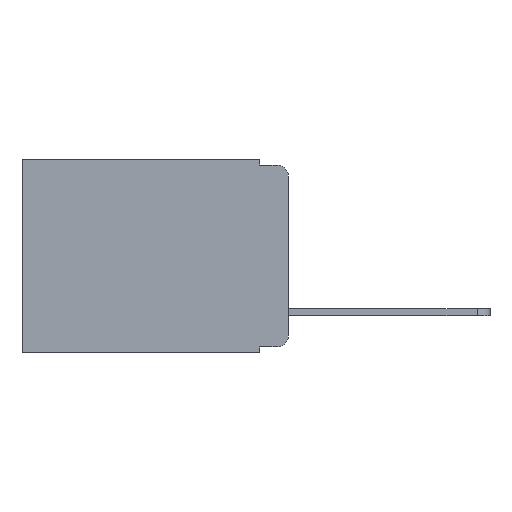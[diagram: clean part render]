
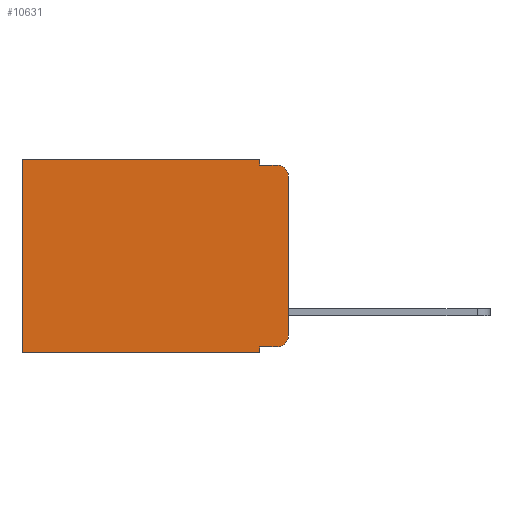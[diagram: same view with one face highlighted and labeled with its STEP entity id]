
A CAD part, left-side view. The second image highlights one B-rep face of the part: STEP entity #10631.
In plain terms, the highlighted planar face has unit normal (-1, 0, 0).
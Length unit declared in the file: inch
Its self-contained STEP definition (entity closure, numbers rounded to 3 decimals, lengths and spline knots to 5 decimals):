
#285 = DIRECTION ( 'NONE',  ( 0., 0., -1. ) ) ;
#680 = VECTOR ( 'NONE', #7780, 39.37008 ) ;
#1125 = ORIENTED_EDGE ( 'NONE', *, *, #13841, .T. ) ;
#1165 = VERTEX_POINT ( 'NONE', #4860 ) ;
#1272 = DIRECTION ( 'NONE',  ( 0., 0., -1. ) ) ;
#1438 = CARTESIAN_POINT ( 'NONE',  ( 0.298, 0.051, 0. ) ) ;
#1664 = VERTEX_POINT ( 'NONE', #4927 ) ;
#1966 = EDGE_LOOP ( 'NONE', ( #3705, #6823, #3880, #10232, #13664, #1125, #7923, #10960, #8287, #14346 ) ) ;
#2559 = DIRECTION ( 'NONE',  ( 1., 0., 0. ) ) ;
#2642 = DIRECTION ( 'NONE',  ( 0., 1., 0. ) ) ;
#3253 = LINE ( 'NONE', #14003, #12418 ) ;
#3318 = EDGE_CURVE ( 'NONE', #4113, #7942, #11637, .T. ) ;
#3705 = ORIENTED_EDGE ( 'NONE', *, *, #4437, .F. ) ;
#3880 = ORIENTED_EDGE ( 'NONE', *, *, #14892, .F. ) ;
#4113 = VERTEX_POINT ( 'NONE', #10030 ) ;
#4163 = EDGE_CURVE ( 'NONE', #7310, #6095, #6894, .T. ) ;
#4204 = VERTEX_POINT ( 'NONE', #15331 ) ;
#4225 = CARTESIAN_POINT ( 'NONE',  ( 0.298, 0., -0.313 ) ) ;
#4250 = CARTESIAN_POINT ( 'NONE',  ( 0.298, 0., -0.03 ) ) ;
#4437 = EDGE_CURVE ( 'NONE', #7310, #7942, #11784, .T. ) ;
#4533 = EDGE_CURVE ( 'NONE', #11388, #5750, #8340, .T. ) ;
#4670 = LINE ( 'NONE', #15644, #13327 ) ;
#4860 = CARTESIAN_POINT ( 'NONE',  ( 0.298, 0.051, -0.01 ) ) ;
#4927 = CARTESIAN_POINT ( 'NONE',  ( 0.298, 0.051, -0.343 ) ) ;
#4986 = CARTESIAN_POINT ( 'NONE',  ( 0.298, 0.02, -0.313 ) ) ;
#5750 = VERTEX_POINT ( 'NONE', #5873 ) ;
#5873 = CARTESIAN_POINT ( 'NONE',  ( 0.298, 0.473, 0. ) ) ;
#6095 = VERTEX_POINT ( 'NONE', #8014 ) ;
#6322 = LINE ( 'NONE', #11859, #15131 ) ;
#6343 = DIRECTION ( 'NONE',  ( -1., 0., 0. ) ) ;
#6374 = PLANE ( 'NONE',  #6998 ) ;
#6377 = CARTESIAN_POINT ( 'NONE',  ( 0.298, 0., 0. ) ) ;
#6823 = ORIENTED_EDGE ( 'NONE', *, *, #4163, .T. ) ;
#6894 = CIRCLE ( 'NONE', #10282, 0.02 ) ;
#6941 = DIRECTION ( 'NONE',  ( 0., 0., -1. ) ) ;
#6998 = AXIS2_PLACEMENT_3D ( 'NONE', #14406, #2559, #11027 ) ;
#7210 = EDGE_CURVE ( 'NONE', #1664, #4204, #4670, .T. ) ;
#7310 = VERTEX_POINT ( 'NONE', #4250 ) ;
#7328 = CARTESIAN_POINT ( 'NONE',  ( 0.298, 0., 0. ) ) ;
#7473 = EDGE_CURVE ( 'NONE', #12283, #1664, #13154, .T. ) ;
#7563 = LINE ( 'NONE', #8011, #13338 ) ;
#7780 = DIRECTION ( 'NONE',  ( 0., 0., -1. ) ) ;
#7923 = ORIENTED_EDGE ( 'NONE', *, *, #7210, .F. ) ;
#7942 = VERTEX_POINT ( 'NONE', #4225 ) ;
#8011 = CARTESIAN_POINT ( 'NONE',  ( 0.298, 0.473, 0. ) ) ;
#8014 = CARTESIAN_POINT ( 'NONE',  ( 0.298, 0.02, -0.01 ) ) ;
#8287 = ORIENTED_EDGE ( 'NONE', *, *, #11092, .T. ) ;
#8340 = LINE ( 'NONE', #7328, #10290 ) ;
#8691 = VECTOR ( 'NONE', #6941, 39.37008 ) ;
#9034 = DIRECTION ( 'NONE',  ( 0., 0., -1. ) ) ;
#9329 = CARTESIAN_POINT ( 'NONE',  ( 0.298, 0.051, 0. ) ) ;
#9593 = DIRECTION ( 'NONE',  ( 0., -1., 0. ) ) ;
#10030 = CARTESIAN_POINT ( 'NONE',  ( 0.298, 0.02, -0.333 ) ) ;
#10232 = ORIENTED_EDGE ( 'NONE', *, *, #14654, .F. ) ;
#10282 = AXIS2_PLACEMENT_3D ( 'NONE', #13014, #15691, #9034 ) ;
#10290 = VECTOR ( 'NONE', #13619, 39.37008 ) ;
#10631 = ADVANCED_FACE ( 'NONE', ( #15462 ), #6374, .F. ) ;
#10960 = ORIENTED_EDGE ( 'NONE', *, *, #7473, .F. ) ;
#11027 = DIRECTION ( 'NONE',  ( 0., 0., -1. ) ) ;
#11092 = EDGE_CURVE ( 'NONE', #12283, #4113, #6322, .T. ) ;
#11388 = VERTEX_POINT ( 'NONE', #14587 ) ;
#11637 = CIRCLE ( 'NONE', #11954, 0.02 ) ;
#11784 = LINE ( 'NONE', #6377, #8691 ) ;
#11859 = CARTESIAN_POINT ( 'NONE',  ( 0.298, 0.051, -0.333 ) ) ;
#11954 = AXIS2_PLACEMENT_3D ( 'NONE', #4986, #6343, #1272 ) ;
#12283 = VERTEX_POINT ( 'NONE', #14046 ) ;
#12418 = VECTOR ( 'NONE', #15116, 39.37008 ) ;
#12812 = VECTOR ( 'NONE', #15068, 39.37008 ) ;
#13014 = CARTESIAN_POINT ( 'NONE',  ( 0.298, 0.02, -0.03 ) ) ;
#13154 = LINE ( 'NONE', #9329, #12812 ) ;
#13327 = VECTOR ( 'NONE', #2642, 39.37008 ) ;
#13338 = VECTOR ( 'NONE', #285, 39.37008 ) ;
#13619 = DIRECTION ( 'NONE',  ( 0., 1., 0. ) ) ;
#13652 = LINE ( 'NONE', #1438, #680 ) ;
#13664 = ORIENTED_EDGE ( 'NONE', *, *, #4533, .T. ) ;
#13841 = EDGE_CURVE ( 'NONE', #5750, #4204, #7563, .T. ) ;
#14003 = CARTESIAN_POINT ( 'NONE',  ( 0.298, 0.051, -0.01 ) ) ;
#14046 = CARTESIAN_POINT ( 'NONE',  ( 0.298, 0.051, -0.333 ) ) ;
#14346 = ORIENTED_EDGE ( 'NONE', *, *, #3318, .T. ) ;
#14406 = CARTESIAN_POINT ( 'NONE',  ( 0.298, 0., 0. ) ) ;
#14587 = CARTESIAN_POINT ( 'NONE',  ( 0.298, 0.051, 0. ) ) ;
#14654 = EDGE_CURVE ( 'NONE', #11388, #1165, #13652, .T. ) ;
#14892 = EDGE_CURVE ( 'NONE', #1165, #6095, #3253, .T. ) ;
#15068 = DIRECTION ( 'NONE',  ( 0., 0., -1. ) ) ;
#15116 = DIRECTION ( 'NONE',  ( 0., -1., 0. ) ) ;
#15131 = VECTOR ( 'NONE', #9593, 39.37008 ) ;
#15331 = CARTESIAN_POINT ( 'NONE',  ( 0.298, 0.473, -0.343 ) ) ;
#15462 = FACE_OUTER_BOUND ( 'NONE', #1966, .T. ) ;
#15644 = CARTESIAN_POINT ( 'NONE',  ( 0.298, 0., -0.343 ) ) ;
#15691 = DIRECTION ( 'NONE',  ( -1., 0., 0. ) ) ;
